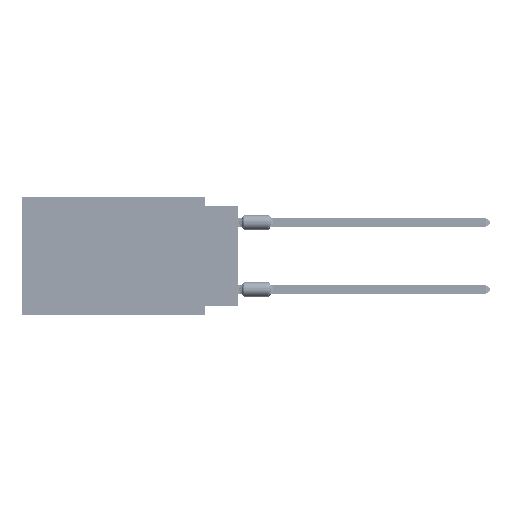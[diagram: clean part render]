
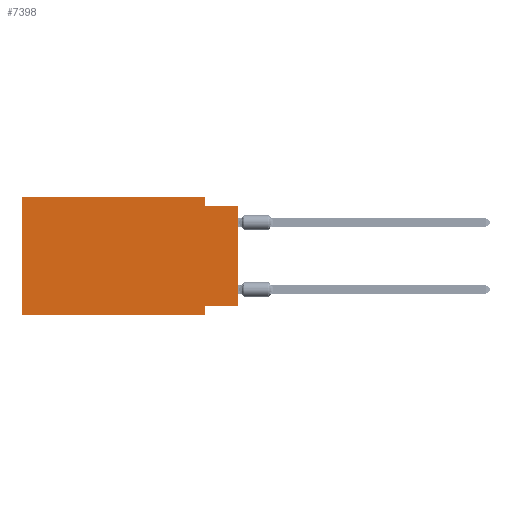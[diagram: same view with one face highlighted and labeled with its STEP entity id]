
A CAD part, left-side view. The second image highlights one B-rep face of the part: STEP entity #7398.
In plain terms, the highlighted planar face has unit normal (-1, 0, 0).
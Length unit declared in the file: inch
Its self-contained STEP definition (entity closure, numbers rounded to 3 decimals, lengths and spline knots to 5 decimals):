
#1476 = LINE ( 'NONE', #108725, #1718 ) ;
#1718 = VECTOR ( 'NONE', #66017, 39.37008 ) ;
#1960 = EDGE_LOOP ( 'NONE', ( #7040, #88217, #64117, #95654, #66068, #89116, #77704, #34242 ) ) ;
#2352 = CARTESIAN_POINT ( 'NONE',  ( 0., 0.645, 0. ) ) ;
#4194 = VERTEX_POINT ( 'NONE', #29695 ) ;
#7040 = ORIENTED_EDGE ( 'NONE', *, *, #40596, .T. ) ;
#7398 = ADVANCED_FACE ( 'NONE', ( #112138 ), #67125, .F. ) ;
#7615 = VERTEX_POINT ( 'NONE', #46134 ) ;
#9799 = LINE ( 'NONE', #80351, #84346 ) ;
#13791 = CARTESIAN_POINT ( 'NONE',  ( 0., 0., -0.325 ) ) ;
#14654 = EDGE_CURVE ( 'NONE', #102462, #58279, #99239, .T. ) ;
#15000 = DIRECTION ( 'NONE',  ( 0., 0., 1. ) ) ;
#15158 = VECTOR ( 'NONE', #114586, 39.37008 ) ;
#16629 = LINE ( 'NONE', #98376, #95495 ) ;
#22913 = CARTESIAN_POINT ( 'NONE',  ( 0., 0., -0.025 ) ) ;
#25532 = DIRECTION ( 'NONE',  ( 0., 0., -1. ) ) ;
#28648 = DIRECTION ( 'NONE',  ( 1., 0., 0. ) ) ;
#29695 = CARTESIAN_POINT ( 'NONE',  ( 0., 0.1, -0.025 ) ) ;
#32832 = LINE ( 'NONE', #41717, #15158 ) ;
#33956 = LINE ( 'NONE', #114546, #36867 ) ;
#34242 = ORIENTED_EDGE ( 'NONE', *, *, #14654, .F. ) ;
#36867 = VECTOR ( 'NONE', #15000, 39.37008 ) ;
#37061 = DIRECTION ( 'NONE',  ( 0., -1., 0. ) ) ;
#38494 = VERTEX_POINT ( 'NONE', #111599 ) ;
#40596 = EDGE_CURVE ( 'NONE', #102462, #7615, #33956, .T. ) ;
#41670 = CARTESIAN_POINT ( 'NONE',  ( 0., 0.645, 0. ) ) ;
#41717 = CARTESIAN_POINT ( 'NONE',  ( 0., 0.1, -0.35 ) ) ;
#45391 = EDGE_CURVE ( 'NONE', #58279, #38494, #32832, .T. ) ;
#46134 = CARTESIAN_POINT ( 'NONE',  ( 0., 0., -0.025 ) ) ;
#47068 = DIRECTION ( 'NONE',  ( 0., 1., 0. ) ) ;
#47364 = LINE ( 'NONE', #2352, #109558 ) ;
#52104 = EDGE_CURVE ( 'NONE', #4194, #7615, #104673, .T. ) ;
#52750 = EDGE_CURVE ( 'NONE', #60870, #4194, #16629, .T. ) ;
#53698 = EDGE_CURVE ( 'NONE', #58725, #38494, #9799, .T. ) ;
#56030 = CARTESIAN_POINT ( 'NONE',  ( 0., 0.1, -0.325 ) ) ;
#56268 = DIRECTION ( 'NONE',  ( 0., -1., 0. ) ) ;
#58279 = VERTEX_POINT ( 'NONE', #56030 ) ;
#58725 = VERTEX_POINT ( 'NONE', #113716 ) ;
#59631 = DIRECTION ( 'NONE',  ( 0., -1., 0. ) ) ;
#60870 = VERTEX_POINT ( 'NONE', #65392 ) ;
#63728 = VECTOR ( 'NONE', #47068, 39.37008 ) ;
#64117 = ORIENTED_EDGE ( 'NONE', *, *, #52750, .F. ) ;
#64576 = AXIS2_PLACEMENT_3D ( 'NONE', #102077, #28648, #103259 ) ;
#65392 = CARTESIAN_POINT ( 'NONE',  ( 0., 0.1, 0. ) ) ;
#66017 = DIRECTION ( 'NONE',  ( 0., 0., 1. ) ) ;
#66068 = ORIENTED_EDGE ( 'NONE', *, *, #108805, .F. ) ;
#67125 = PLANE ( 'NONE',  #64576 ) ;
#69414 = EDGE_CURVE ( 'NONE', #87517, #60870, #47364, .T. ) ;
#77704 = ORIENTED_EDGE ( 'NONE', *, *, #45391, .F. ) ;
#80351 = CARTESIAN_POINT ( 'NONE',  ( 0., 0.645, -0.35 ) ) ;
#84089 = VECTOR ( 'NONE', #59631, 39.37008 ) ;
#84346 = VECTOR ( 'NONE', #37061, 39.37008 ) ;
#87517 = VERTEX_POINT ( 'NONE', #41670 ) ;
#88217 = ORIENTED_EDGE ( 'NONE', *, *, #52104, .F. ) ;
#89116 = ORIENTED_EDGE ( 'NONE', *, *, #53698, .T. ) ;
#95495 = VECTOR ( 'NONE', #25532, 39.37008 ) ;
#95654 = ORIENTED_EDGE ( 'NONE', *, *, #69414, .F. ) ;
#98376 = CARTESIAN_POINT ( 'NONE',  ( 0., 0.1, 0. ) ) ;
#99239 = LINE ( 'NONE', #100985, #63728 ) ;
#100985 = CARTESIAN_POINT ( 'NONE',  ( 0., 0., -0.325 ) ) ;
#102077 = CARTESIAN_POINT ( 'NONE',  ( 0., 0.645, 0. ) ) ;
#102462 = VERTEX_POINT ( 'NONE', #13791 ) ;
#103259 = DIRECTION ( 'NONE',  ( 0., 0., -1. ) ) ;
#104673 = LINE ( 'NONE', #22913, #84089 ) ;
#108725 = CARTESIAN_POINT ( 'NONE',  ( 0., 0.645, 0. ) ) ;
#108805 = EDGE_CURVE ( 'NONE', #58725, #87517, #1476, .T. ) ;
#109558 = VECTOR ( 'NONE', #56268, 39.37008 ) ;
#111599 = CARTESIAN_POINT ( 'NONE',  ( 0., 0.1, -0.35 ) ) ;
#112138 = FACE_OUTER_BOUND ( 'NONE', #1960, .T. ) ;
#113716 = CARTESIAN_POINT ( 'NONE',  ( 0., 0.645, -0.35 ) ) ;
#114546 = CARTESIAN_POINT ( 'NONE',  ( 0., 0., 0. ) ) ;
#114586 = DIRECTION ( 'NONE',  ( 0., 0., -1. ) ) ;
